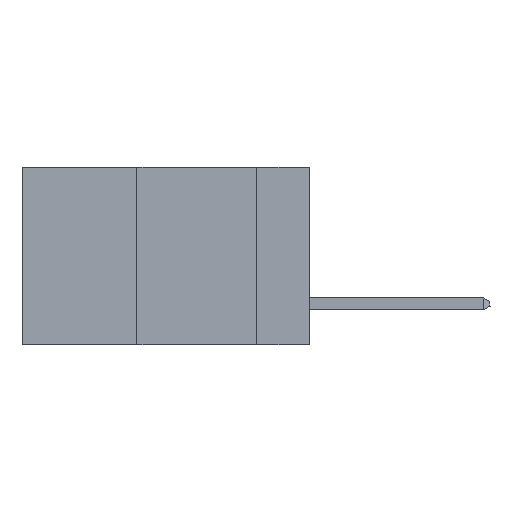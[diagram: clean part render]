
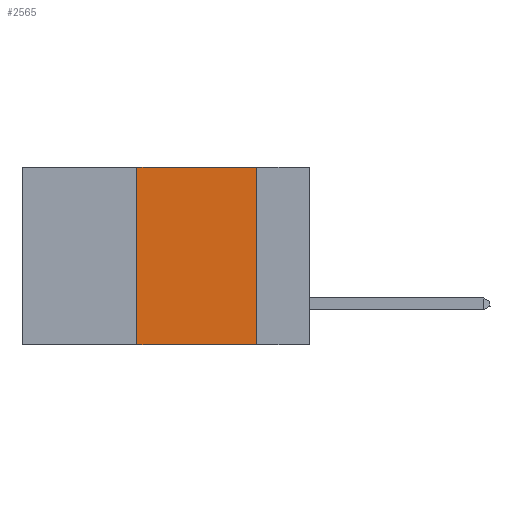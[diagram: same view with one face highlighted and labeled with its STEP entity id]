
A CAD part, left-side view. The second image highlights one B-rep face of the part: STEP entity #2565.
In plain terms, the highlighted planar face has unit normal (-1, 0, 0).
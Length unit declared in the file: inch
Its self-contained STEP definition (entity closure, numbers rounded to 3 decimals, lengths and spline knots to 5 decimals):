
#434 = DIRECTION ( 'NONE',  ( 0., 0., -1. ) ) ;
#590 = CARTESIAN_POINT ( 'NONE',  ( 0., 0.11, -0.37 ) ) ;
#1175 = CARTESIAN_POINT ( 'NONE',  ( 0., 0.36, -0.37 ) ) ;
#1826 = CARTESIAN_POINT ( 'NONE',  ( 0., 0.6, -0.37 ) ) ;
#2565 = ADVANCED_FACE ( 'NONE', ( #11817 ), #16473, .F. ) ;
#3246 = ORIENTED_EDGE ( 'NONE', *, *, #21303, .T. ) ;
#4228 = VECTOR ( 'NONE', #11852, 39.37008 ) ;
#4399 = CARTESIAN_POINT ( 'NONE',  ( 0., 0.6, 0. ) ) ;
#4632 = DIRECTION ( 'NONE',  ( 0., -1., 0. ) ) ;
#4670 = VECTOR ( 'NONE', #4632, 39.37008 ) ;
#5332 = VERTEX_POINT ( 'NONE', #23138 ) ;
#5515 = VERTEX_POINT ( 'NONE', #1175 ) ;
#6811 = ORIENTED_EDGE ( 'NONE', *, *, #21325, .F. ) ;
#6970 = LINE ( 'NONE', #7931, #18976 ) ;
#7931 = CARTESIAN_POINT ( 'NONE',  ( 0., 0.36, 0. ) ) ;
#8164 = EDGE_LOOP ( 'NONE', ( #6811, #10389, #14352, #3246 ) ) ;
#9461 = EDGE_CURVE ( 'NONE', #5515, #5332, #6970, .T. ) ;
#9617 = VECTOR ( 'NONE', #11680, 39.37008 ) ;
#10389 = ORIENTED_EDGE ( 'NONE', *, *, #12231, .F. ) ;
#10638 = VERTEX_POINT ( 'NONE', #13828 ) ;
#11642 = LINE ( 'NONE', #18910, #4670 ) ;
#11680 = DIRECTION ( 'NONE',  ( 0., 0., -1. ) ) ;
#11817 = FACE_OUTER_BOUND ( 'NONE', #8164, .T. ) ;
#11852 = DIRECTION ( 'NONE',  ( 0., -1., 0. ) ) ;
#12042 = VERTEX_POINT ( 'NONE', #590 ) ;
#12231 = EDGE_CURVE ( 'NONE', #5332, #10638, #11642, .T. ) ;
#12513 = DIRECTION ( 'NONE',  ( 1., 0., 0. ) ) ;
#13594 = AXIS2_PLACEMENT_3D ( 'NONE', #4399, #12513, #434 ) ;
#13828 = CARTESIAN_POINT ( 'NONE',  ( 0., 0.11, 0. ) ) ;
#14352 = ORIENTED_EDGE ( 'NONE', *, *, #9461, .F. ) ;
#14945 = LINE ( 'NONE', #21631, #9617 ) ;
#16473 = PLANE ( 'NONE',  #13594 ) ;
#18910 = CARTESIAN_POINT ( 'NONE',  ( 0., 0.6, 0. ) ) ;
#18976 = VECTOR ( 'NONE', #20340, 39.37008 ) ;
#20340 = DIRECTION ( 'NONE',  ( 0., 0., 1. ) ) ;
#20629 = LINE ( 'NONE', #1826, #4228 ) ;
#21303 = EDGE_CURVE ( 'NONE', #5515, #12042, #20629, .T. ) ;
#21325 = EDGE_CURVE ( 'NONE', #10638, #12042, #14945, .T. ) ;
#21631 = CARTESIAN_POINT ( 'NONE',  ( 0., 0.11, 0. ) ) ;
#23138 = CARTESIAN_POINT ( 'NONE',  ( 0., 0.36, 0. ) ) ;
